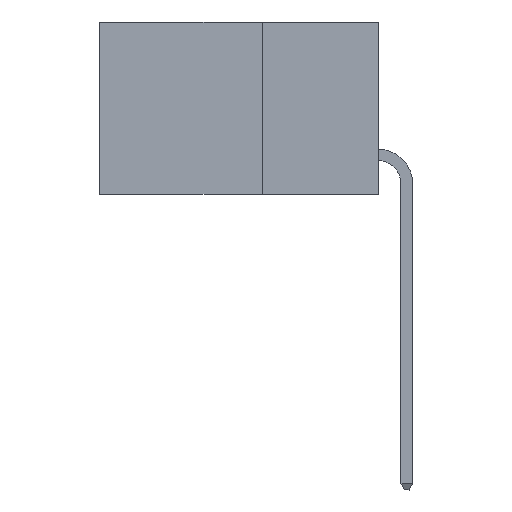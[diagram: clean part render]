
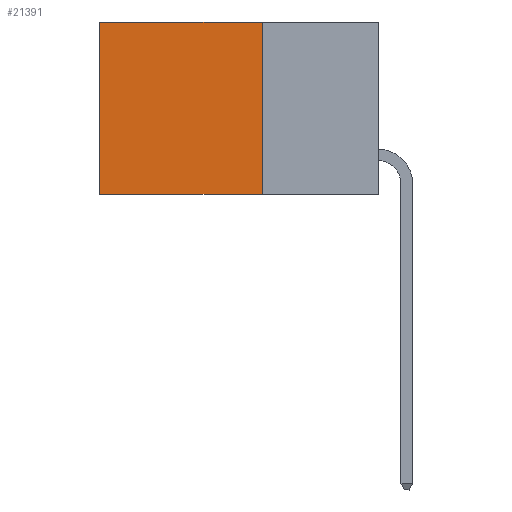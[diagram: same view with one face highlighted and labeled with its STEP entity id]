
A CAD part, left-side view. The second image highlights one B-rep face of the part: STEP entity #21391.
In plain terms, the highlighted planar face has unit normal (-1, 0, 0).
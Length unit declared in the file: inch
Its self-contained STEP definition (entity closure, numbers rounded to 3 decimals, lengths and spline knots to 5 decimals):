
#62 = CARTESIAN_POINT ( 'NONE',  ( 0.298, 0.25, -0.37 ) ) ;
#924 = PLANE ( 'NONE',  #10016 ) ;
#3304 = DIRECTION ( 'NONE',  ( 0., 0., -1. ) ) ;
#3436 = CARTESIAN_POINT ( 'NONE',  ( 0.298, 0.25, 0. ) ) ;
#3699 = VERTEX_POINT ( 'NONE', #23211 ) ;
#4245 = VERTEX_POINT ( 'NONE', #62 ) ;
#4325 = EDGE_CURVE ( 'NONE', #21865, #4245, #25631, .T. ) ;
#4460 = CARTESIAN_POINT ( 'NONE',  ( 0.298, 0.6, 0. ) ) ;
#4862 = EDGE_CURVE ( 'NONE', #7115, #3699, #6526, .T. ) ;
#5232 = DIRECTION ( 'NONE',  ( 0., 0., -1. ) ) ;
#6226 = VECTOR ( 'NONE', #22784, 39.37008 ) ;
#6526 = LINE ( 'NONE', #4460, #23640 ) ;
#7115 = VERTEX_POINT ( 'NONE', #23023 ) ;
#9933 = VECTOR ( 'NONE', #24712, 39.37008 ) ;
#10016 = AXIS2_PLACEMENT_3D ( 'NONE', #15996, #18221, #5232 ) ;
#10697 = ORIENTED_EDGE ( 'NONE', *, *, #4862, .T. ) ;
#12686 = LINE ( 'NONE', #3436, #6226 ) ;
#13576 = ORIENTED_EDGE ( 'NONE', *, *, #16666, .T. ) ;
#14215 = LINE ( 'NONE', #26326, #24834 ) ;
#15996 = CARTESIAN_POINT ( 'NONE',  ( 0.298, 0.25, 0. ) ) ;
#16666 = EDGE_CURVE ( 'NONE', #21865, #7115, #12686, .T. ) ;
#17658 = ORIENTED_EDGE ( 'NONE', *, *, #19990, .F. ) ;
#17973 = DIRECTION ( 'NONE',  ( 0., 1., 0. ) ) ;
#18221 = DIRECTION ( 'NONE',  ( 1., 0., 0. ) ) ;
#18253 = ORIENTED_EDGE ( 'NONE', *, *, #4325, .F. ) ;
#19990 = EDGE_CURVE ( 'NONE', #4245, #3699, #14215, .T. ) ;
#20145 = FACE_OUTER_BOUND ( 'NONE', #21006, .T. ) ;
#21006 = EDGE_LOOP ( 'NONE', ( #10697, #17658, #18253, #13576 ) ) ;
#21391 = ADVANCED_FACE ( 'NONE', ( #20145 ), #924, .F. ) ;
#21760 = CARTESIAN_POINT ( 'NONE',  ( 0.298, 0.25, 0. ) ) ;
#21865 = VERTEX_POINT ( 'NONE', #21760 ) ;
#22784 = DIRECTION ( 'NONE',  ( 0., 1., 0. ) ) ;
#23023 = CARTESIAN_POINT ( 'NONE',  ( 0.298, 0.6, 0. ) ) ;
#23211 = CARTESIAN_POINT ( 'NONE',  ( 0.298, 0.6, -0.37 ) ) ;
#23325 = CARTESIAN_POINT ( 'NONE',  ( 0.298, 0.25, 0. ) ) ;
#23640 = VECTOR ( 'NONE', #3304, 39.37008 ) ;
#24712 = DIRECTION ( 'NONE',  ( 0., 0., -1. ) ) ;
#24834 = VECTOR ( 'NONE', #17973, 39.37008 ) ;
#25631 = LINE ( 'NONE', #23325, #9933 ) ;
#26326 = CARTESIAN_POINT ( 'NONE',  ( 0.298, 0.25, -0.37 ) ) ;
